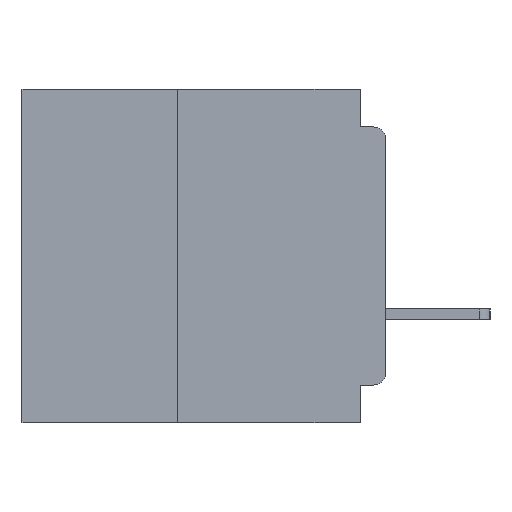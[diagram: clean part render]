
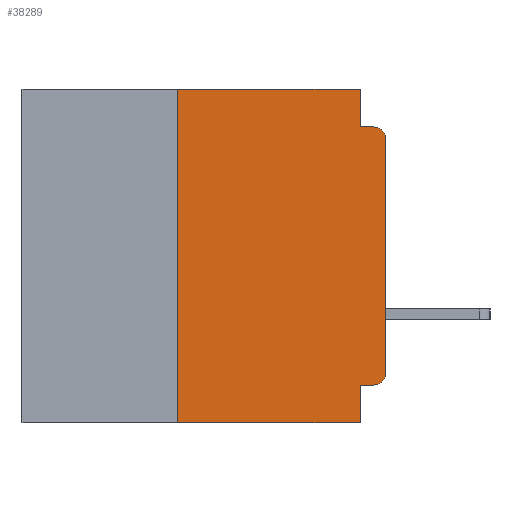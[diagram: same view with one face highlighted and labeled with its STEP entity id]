
A CAD part, left-side view. The second image highlights one B-rep face of the part: STEP entity #38289.
In plain terms, the highlighted planar face has unit normal (-1, 0, 0).
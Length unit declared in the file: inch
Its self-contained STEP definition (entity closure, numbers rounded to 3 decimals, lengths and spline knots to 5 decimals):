
#348 = CARTESIAN_POINT ( 'NONE',  ( 0., 0., 0. ) ) ;
#449 = VERTEX_POINT ( 'NONE', #36033 ) ;
#1017 = CARTESIAN_POINT ( 'NONE',  ( 0., 0.031, 0. ) ) ;
#1780 = CARTESIAN_POINT ( 'NONE',  ( 0., 0.25, -0.4 ) ) ;
#2370 = VECTOR ( 'NONE', #27601, 39.37008 ) ;
#2380 = CARTESIAN_POINT ( 'NONE',  ( 0., 0.031, -0.355 ) ) ;
#2431 = CARTESIAN_POINT ( 'NONE',  ( 0., 0.015, -0.06 ) ) ;
#2844 = EDGE_CURVE ( 'NONE', #46253, #4435, #37883, .T. ) ;
#3482 = DIRECTION ( 'NONE',  ( 1., 0., 0. ) ) ;
#3628 = AXIS2_PLACEMENT_3D ( 'NONE', #2431, #32586, #6821 ) ;
#4435 = VERTEX_POINT ( 'NONE', #1017 ) ;
#4558 = CARTESIAN_POINT ( 'NONE',  ( 0., 0.031, -0.045 ) ) ;
#4897 = VECTOR ( 'NONE', #43680, 39.37008 ) ;
#4939 = VERTEX_POINT ( 'NONE', #43727 ) ;
#5962 = CARTESIAN_POINT ( 'NONE',  ( 0., 0., -0.355 ) ) ;
#6165 = DIRECTION ( 'NONE',  ( 0., 0., 1. ) ) ;
#6570 = VECTOR ( 'NONE', #45314, 39.37008 ) ;
#6821 = DIRECTION ( 'NONE',  ( 0., 0., -1. ) ) ;
#7085 = CARTESIAN_POINT ( 'NONE',  ( 0., 0.437, -0.4 ) ) ;
#7779 = DIRECTION ( 'NONE',  ( -1., 0., 0. ) ) ;
#10029 = CARTESIAN_POINT ( 'NONE',  ( 0., 0.015, -0.355 ) ) ;
#10154 = ORIENTED_EDGE ( 'NONE', *, *, #17017, .F. ) ;
#10965 = CARTESIAN_POINT ( 'NONE',  ( 0., 0.031, 0. ) ) ;
#11513 = ORIENTED_EDGE ( 'NONE', *, *, #19377, .T. ) ;
#13829 = CARTESIAN_POINT ( 'NONE',  ( 0., 0., -0.045 ) ) ;
#13986 = EDGE_CURVE ( 'NONE', #4435, #35018, #17969, .T. ) ;
#15511 = AXIS2_PLACEMENT_3D ( 'NONE', #33540, #7779, #37847 ) ;
#17017 = EDGE_CURVE ( 'NONE', #35018, #28717, #51459, .T. ) ;
#17091 = ORIENTED_EDGE ( 'NONE', *, *, #18563, .F. ) ;
#17118 = LINE ( 'NONE', #45605, #27225 ) ;
#17919 = VERTEX_POINT ( 'NONE', #45477 ) ;
#17969 = LINE ( 'NONE', #10965, #6570 ) ;
#18128 = DIRECTION ( 'NONE',  ( 0., -1., 0. ) ) ;
#18563 = EDGE_CURVE ( 'NONE', #35841, #17919, #17118, .T. ) ;
#19377 = EDGE_CURVE ( 'NONE', #449, #28816, #39885, .T. ) ;
#19847 = DIRECTION ( 'NONE',  ( 0., 0., -1. ) ) ;
#20586 = CARTESIAN_POINT ( 'NONE',  ( 0., 0.437, 0. ) ) ;
#21762 = VECTOR ( 'NONE', #24358, 39.37008 ) ;
#24358 = DIRECTION ( 'NONE',  ( 0., -1., 0. ) ) ;
#24905 = PLANE ( 'NONE',  #55244 ) ;
#25275 = LINE ( 'NONE', #5962, #2370 ) ;
#26411 = CIRCLE ( 'NONE', #3628, 0.015 ) ;
#27225 = VECTOR ( 'NONE', #19847, 39.37008 ) ;
#27601 = DIRECTION ( 'NONE',  ( 0., 1., 0. ) ) ;
#28489 = VECTOR ( 'NONE', #47556, 39.37008 ) ;
#28555 = ORIENTED_EDGE ( 'NONE', *, *, #53307, .T. ) ;
#28717 = VERTEX_POINT ( 'NONE', #31710 ) ;
#28816 = VERTEX_POINT ( 'NONE', #36753 ) ;
#29975 = EDGE_CURVE ( 'NONE', #4939, #46253, #44724, .T. ) ;
#31710 = CARTESIAN_POINT ( 'NONE',  ( 0., 0.015, -0.045 ) ) ;
#32586 = DIRECTION ( 'NONE',  ( -1., 0., 0. ) ) ;
#33258 = LINE ( 'NONE', #7085, #21762 ) ;
#33353 = VECTOR ( 'NONE', #6165, 39.37008 ) ;
#33540 = CARTESIAN_POINT ( 'NONE',  ( 0., 0.015, -0.34 ) ) ;
#33588 = DIRECTION ( 'NONE',  ( 0., 0., -1. ) ) ;
#33694 = EDGE_CURVE ( 'NONE', #28816, #28717, #26411, .T. ) ;
#35018 = VERTEX_POINT ( 'NONE', #4558 ) ;
#35841 = VERTEX_POINT ( 'NONE', #2380 ) ;
#36033 = CARTESIAN_POINT ( 'NONE',  ( 0., 0., -0.34 ) ) ;
#36753 = CARTESIAN_POINT ( 'NONE',  ( 0., 0., -0.06 ) ) ;
#37435 = CARTESIAN_POINT ( 'NONE',  ( 0., 0.25, 0. ) ) ;
#37847 = DIRECTION ( 'NONE',  ( 0., 0., -1. ) ) ;
#37883 = LINE ( 'NONE', #43994, #4897 ) ;
#38045 = EDGE_CURVE ( 'NONE', #40408, #35841, #25275, .T. ) ;
#38289 = ADVANCED_FACE ( 'NONE', ( #46087 ), #24905, .F. ) ;
#39637 = ORIENTED_EDGE ( 'NONE', *, *, #29975, .F. ) ;
#39885 = LINE ( 'NONE', #348, #28489 ) ;
#40088 = VECTOR ( 'NONE', #18128, 39.37008 ) ;
#40408 = VERTEX_POINT ( 'NONE', #10029 ) ;
#41621 = ORIENTED_EDGE ( 'NONE', *, *, #38045, .F. ) ;
#42037 = ORIENTED_EDGE ( 'NONE', *, *, #33694, .T. ) ;
#43680 = DIRECTION ( 'NONE',  ( 0., -1., 0. ) ) ;
#43727 = CARTESIAN_POINT ( 'NONE',  ( 0., 0.25, -0.4 ) ) ;
#43994 = CARTESIAN_POINT ( 'NONE',  ( 0., 0.437, 0. ) ) ;
#44724 = LINE ( 'NONE', #1780, #33353 ) ;
#45314 = DIRECTION ( 'NONE',  ( 0., 0., -1. ) ) ;
#45477 = CARTESIAN_POINT ( 'NONE',  ( 0., 0.031, -0.4 ) ) ;
#45605 = CARTESIAN_POINT ( 'NONE',  ( 0., 0.031, -0.4 ) ) ;
#46087 = FACE_OUTER_BOUND ( 'NONE', #51754, .T. ) ;
#46219 = ORIENTED_EDGE ( 'NONE', *, *, #13986, .F. ) ;
#46253 = VERTEX_POINT ( 'NONE', #37435 ) ;
#46912 = ORIENTED_EDGE ( 'NONE', *, *, #2844, .F. ) ;
#47556 = DIRECTION ( 'NONE',  ( 0., 0., 1. ) ) ;
#49140 = ORIENTED_EDGE ( 'NONE', *, *, #50815, .T. ) ;
#49666 = CIRCLE ( 'NONE', #15511, 0.015 ) ;
#50815 = EDGE_CURVE ( 'NONE', #4939, #17919, #33258, .T. ) ;
#51459 = LINE ( 'NONE', #13829, #40088 ) ;
#51754 = EDGE_LOOP ( 'NONE', ( #11513, #42037, #10154, #46219, #46912, #39637, #49140, #17091, #41621, #28555 ) ) ;
#53307 = EDGE_CURVE ( 'NONE', #40408, #449, #49666, .T. ) ;
#55244 = AXIS2_PLACEMENT_3D ( 'NONE', #20586, #3482, #33588 ) ;
